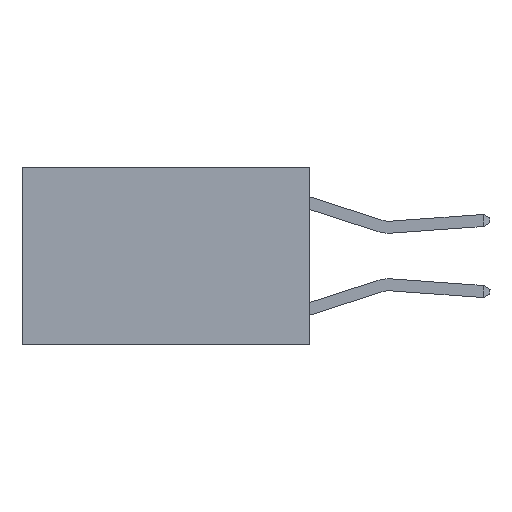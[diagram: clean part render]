
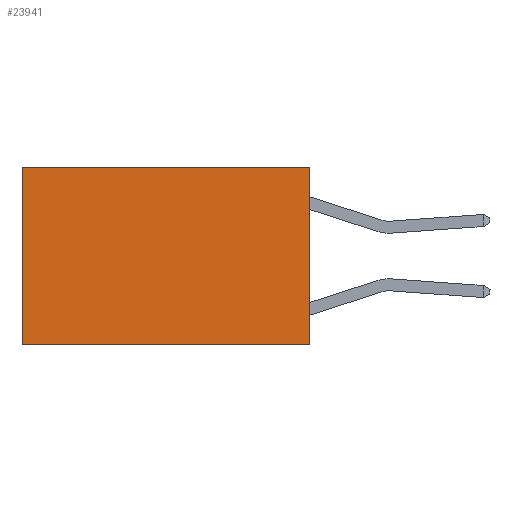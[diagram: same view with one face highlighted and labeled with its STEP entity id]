
A CAD part, left-side view. The second image highlights one B-rep face of the part: STEP entity #23941.
In plain terms, the highlighted planar face has unit normal (-1, 0, 0).
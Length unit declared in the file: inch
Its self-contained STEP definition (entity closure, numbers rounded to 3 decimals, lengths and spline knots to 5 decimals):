
#25 = EDGE_CURVE ( 'NONE', #22640, #9113, #16424, .T. ) ;
#541 = CARTESIAN_POINT ( 'NONE',  ( 0.2625, 0.6, -0.37 ) ) ;
#724 = FACE_OUTER_BOUND ( 'NONE', #2894, .T. ) ;
#2534 = CARTESIAN_POINT ( 'NONE',  ( 0.2625, 0., -0.37 ) ) ;
#2651 = VECTOR ( 'NONE', #11788, 39.37008 ) ;
#2894 = EDGE_LOOP ( 'NONE', ( #23076, #8627, #9703, #22889 ) ) ;
#2914 = EDGE_CURVE ( 'NONE', #20368, #3062, #3546, .T. ) ;
#2984 = PLANE ( 'NONE',  #4183 ) ;
#3062 = VERTEX_POINT ( 'NONE', #11728 ) ;
#3546 = LINE ( 'NONE', #18084, #22609 ) ;
#4183 = AXIS2_PLACEMENT_3D ( 'NONE', #19956, #4884, #18228 ) ;
#4884 = DIRECTION ( 'NONE',  ( 1., 0., 0. ) ) ;
#6149 = CARTESIAN_POINT ( 'NONE',  ( 0.2625, 0., -0.37 ) ) ;
#7877 = VECTOR ( 'NONE', #9982, 39.37008 ) ;
#8212 = CARTESIAN_POINT ( 'NONE',  ( 0.2625, 0.6, 0. ) ) ;
#8627 = ORIENTED_EDGE ( 'NONE', *, *, #25, .F. ) ;
#9113 = VERTEX_POINT ( 'NONE', #541 ) ;
#9703 = ORIENTED_EDGE ( 'NONE', *, *, #17118, .F. ) ;
#9982 = DIRECTION ( 'NONE',  ( 0., 0., -1. ) ) ;
#10051 = DIRECTION ( 'NONE',  ( 0., 1., 0. ) ) ;
#11728 = CARTESIAN_POINT ( 'NONE',  ( 0.2625, 0.6, 0. ) ) ;
#11788 = DIRECTION ( 'NONE',  ( 0., 0., -1. ) ) ;
#16424 = LINE ( 'NONE', #6149, #20864 ) ;
#17118 = EDGE_CURVE ( 'NONE', #20368, #22640, #17271, .T. ) ;
#17271 = LINE ( 'NONE', #23232, #2651 ) ;
#18084 = CARTESIAN_POINT ( 'NONE',  ( 0.2625, 0., 0. ) ) ;
#18228 = DIRECTION ( 'NONE',  ( 0., 0., -1. ) ) ;
#18646 = EDGE_CURVE ( 'NONE', #3062, #9113, #23133, .T. ) ;
#19294 = CARTESIAN_POINT ( 'NONE',  ( 0.2625, 0., 0. ) ) ;
#19956 = CARTESIAN_POINT ( 'NONE',  ( 0.2625, 0., 0. ) ) ;
#20368 = VERTEX_POINT ( 'NONE', #19294 ) ;
#20864 = VECTOR ( 'NONE', #24536, 39.37008 ) ;
#22609 = VECTOR ( 'NONE', #10051, 39.37008 ) ;
#22640 = VERTEX_POINT ( 'NONE', #2534 ) ;
#22889 = ORIENTED_EDGE ( 'NONE', *, *, #2914, .T. ) ;
#23076 = ORIENTED_EDGE ( 'NONE', *, *, #18646, .T. ) ;
#23133 = LINE ( 'NONE', #8212, #7877 ) ;
#23232 = CARTESIAN_POINT ( 'NONE',  ( 0.2625, 0., 0. ) ) ;
#23941 = ADVANCED_FACE ( 'NONE', ( #724 ), #2984, .F. ) ;
#24536 = DIRECTION ( 'NONE',  ( 0., 1., 0. ) ) ;
